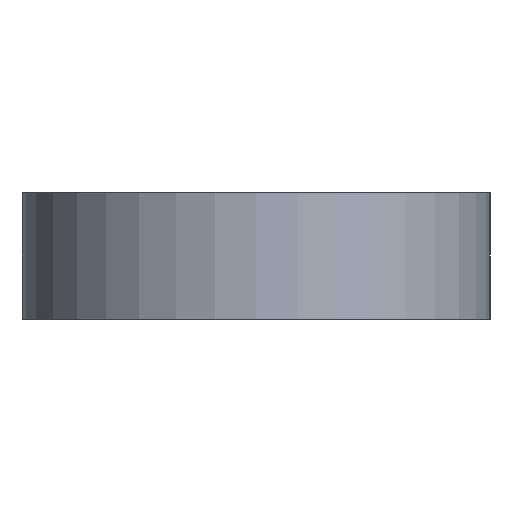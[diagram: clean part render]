
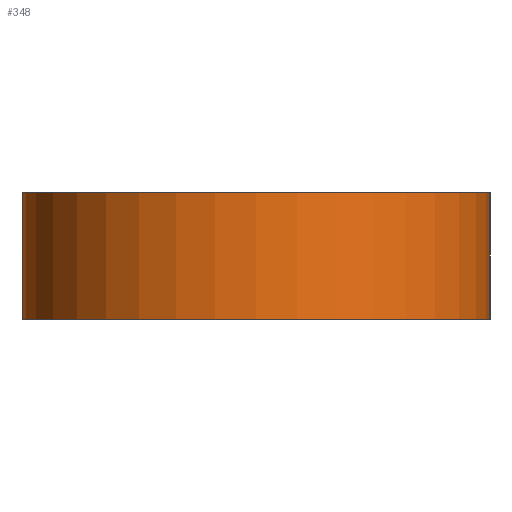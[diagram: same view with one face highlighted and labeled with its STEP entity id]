
A CAD part, front view. The second image highlights one B-rep face of the part: STEP entity #348.
In plain terms, the highlighted cylindrical face has radius 18.567 mm (diameter 37.133 mm), a partial arc.
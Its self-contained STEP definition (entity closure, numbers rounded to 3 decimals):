
#16 = CYLINDRICAL_SURFACE ( 'NONE', #33, 18.567 ) ;
#28 = FACE_OUTER_BOUND ( 'NONE', #133, .T. ) ;
#33 = AXIS2_PLACEMENT_3D ( 'NONE', #191, #208, #195 ) ;
#53 = VECTOR ( 'NONE', #269, 1000. ) ;
#56 = VECTOR ( 'NONE', #311, 1000. ) ;
#57 = LINE ( 'NONE', #271, #53 ) ;
#59 = LINE ( 'NONE', #272, #56 ) ;
#61 = CIRCLE ( 'NONE', #172, 18.567 ) ;
#78 = CIRCLE ( 'NONE', #120, 18.567 ) ;
#96 = EDGE_CURVE ( 'NONE', #119, #117, #78, .T. ) ;
#100 = EDGE_CURVE ( 'NONE', #114, #119, #59, .T. ) ;
#101 = EDGE_CURVE ( 'NONE', #115, #117, #57, .T. ) ;
#102 = EDGE_CURVE ( 'NONE', #114, #115, #61, .T. ) ;
#105 = ORIENTED_EDGE ( 'NONE', *, *, #102, .F. ) ;
#114 = VERTEX_POINT ( 'NONE', #233 ) ;
#115 = VERTEX_POINT ( 'NONE', #261 ) ;
#117 = VERTEX_POINT ( 'NONE', #240 ) ;
#119 = VERTEX_POINT ( 'NONE', #202 ) ;
#120 = AXIS2_PLACEMENT_3D ( 'NONE', #314, #313, #312 ) ;
#127 = ORIENTED_EDGE ( 'NONE', *, *, #101, .F. ) ;
#132 = ORIENTED_EDGE ( 'NONE', *, *, #96, .T. ) ;
#133 = EDGE_LOOP ( 'NONE', ( #132, #127, #105, #327 ) ) ;
#172 = AXIS2_PLACEMENT_3D ( 'NONE', #267, #255, #265 ) ;
#191 = CARTESIAN_POINT ( 'NONE',  ( 0.012, -88.078, 10. ) ) ;
#195 = DIRECTION ( 'NONE',  ( -1., 0., 0. ) ) ;
#202 = CARTESIAN_POINT ( 'NONE',  ( -18.555, -88.078, 0. ) ) ;
#208 = DIRECTION ( 'NONE',  ( 0., 0., -1. ) ) ;
#233 = CARTESIAN_POINT ( 'NONE',  ( -18.555, -88.078, 10. ) ) ;
#240 = CARTESIAN_POINT ( 'NONE',  ( 18.578, -88.078, 0. ) ) ;
#255 = DIRECTION ( 'NONE',  ( 0., 0., 1. ) ) ;
#261 = CARTESIAN_POINT ( 'NONE',  ( 18.578, -88.078, 10. ) ) ;
#265 = DIRECTION ( 'NONE',  ( 1., 0., 0. ) ) ;
#267 = CARTESIAN_POINT ( 'NONE',  ( 0.012, -88.078, 10. ) ) ;
#269 = DIRECTION ( 'NONE',  ( 0., 0., -1. ) ) ;
#271 = CARTESIAN_POINT ( 'NONE',  ( 18.578, -88.078, 10. ) ) ;
#272 = CARTESIAN_POINT ( 'NONE',  ( -18.555, -88.078, 10. ) ) ;
#311 = DIRECTION ( 'NONE',  ( 0., 0., -1. ) ) ;
#312 = DIRECTION ( 'NONE',  ( 1., 0., 0. ) ) ;
#313 = DIRECTION ( 'NONE',  ( 0., 0., 1. ) ) ;
#314 = CARTESIAN_POINT ( 'NONE',  ( 0.012, -88.078, 0. ) ) ;
#327 = ORIENTED_EDGE ( 'NONE', *, *, #100, .T. ) ;
#348 = ADVANCED_FACE ( 'NONE', ( #28 ), #16, .T. ) ;
